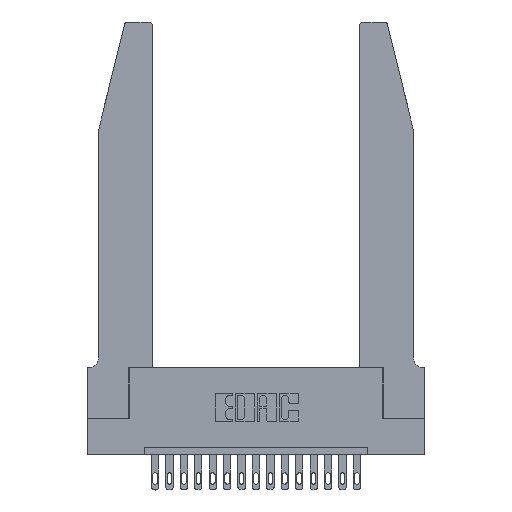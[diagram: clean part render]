
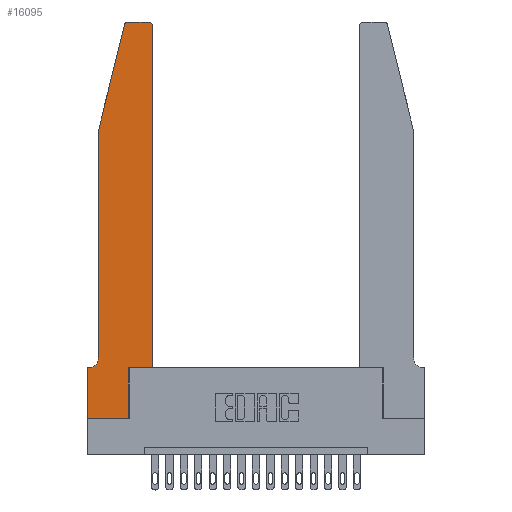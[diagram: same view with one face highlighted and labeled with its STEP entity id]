
A CAD part, top view. The second image highlights one B-rep face of the part: STEP entity #16095.
In plain terms, the highlighted planar face has unit normal (0, 0, 1).
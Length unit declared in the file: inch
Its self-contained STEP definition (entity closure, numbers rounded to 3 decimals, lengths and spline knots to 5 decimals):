
#24 = DIRECTION ( 'NONE',  ( 1., 0., 0. ) ) ;
#91 = DIRECTION ( 'NONE',  ( 0., 1., 0. ) ) ;
#96 = VECTOR ( 'NONE', #12066, 39.37008 ) ;
#188 = VECTOR ( 'NONE', #8749, 39.37008 ) ;
#674 = VECTOR ( 'NONE', #91, 39.37008 ) ;
#808 = CARTESIAN_POINT ( 'NONE',  ( 0.4505, 0.35, 0.37 ) ) ;
#891 = ORIENTED_EDGE ( 'NONE', *, *, #6180, .T. ) ;
#1024 = EDGE_CURVE ( 'NONE', #6409, #7204, #5909, .T. ) ;
#1132 = DIRECTION ( 'NONE',  ( 0., 0., 1. ) ) ;
#1140 = CARTESIAN_POINT ( 'NONE',  ( 0., 0.35, 0.37 ) ) ;
#1428 = VERTEX_POINT ( 'NONE', #13695 ) ;
#1525 = ORIENTED_EDGE ( 'NONE', *, *, #14287, .T. ) ;
#1633 = CARTESIAN_POINT ( 'NONE',  ( 0.2865, 0.35, 0.37 ) ) ;
#1952 = ORIENTED_EDGE ( 'NONE', *, *, #12184, .T. ) ;
#2261 = AXIS2_PLACEMENT_3D ( 'NONE', #11477, #1132, #11677 ) ;
#2593 = CARTESIAN_POINT ( 'NONE',  ( 0.0055, 0.35, 0.37 ) ) ;
#2756 = CIRCLE ( 'NONE', #7343, 0.03 ) ;
#2979 = CARTESIAN_POINT ( 'NONE',  ( 0.0755, 2., 0.37 ) ) ;
#3049 = EDGE_CURVE ( 'NONE', #4441, #1428, #5342, .T. ) ;
#3478 = CARTESIAN_POINT ( 'NONE',  ( 0.0755, 2., 0.37 ) ) ;
#3557 = LINE ( 'NONE', #12129, #8222 ) ;
#3671 = CARTESIAN_POINT ( 'NONE',  ( 0.284, 2.75, 0.37 ) ) ;
#3723 = DIRECTION ( 'NONE',  ( -1., 0., 0. ) ) ;
#3912 = CARTESIAN_POINT ( 'NONE',  ( 0.0755, 2., 0.37 ) ) ;
#3958 = LINE ( 'NONE', #9079, #674 ) ;
#4337 = VERTEX_POINT ( 'NONE', #14523 ) ;
#4441 = VERTEX_POINT ( 'NONE', #6452 ) ;
#4548 = LINE ( 'NONE', #15057, #96 ) ;
#4711 = EDGE_CURVE ( 'NONE', #12307, #4441, #3557, .T. ) ;
#5292 = CARTESIAN_POINT ( 'NONE',  ( 0.2605, 2.75, 0.37 ) ) ;
#5342 = LINE ( 'NONE', #6000, #188 ) ;
#5587 = AXIS2_PLACEMENT_3D ( 'NONE', #15855, #12849, #13053 ) ;
#5701 = ORIENTED_EDGE ( 'NONE', *, *, #3049, .T. ) ;
#5909 = CIRCLE ( 'NONE', #2261, 0.03 ) ;
#6000 = CARTESIAN_POINT ( 'NONE',  ( 0., 0., 0.37 ) ) ;
#6035 = EDGE_CURVE ( 'NONE', #13699, #18647, #12219, .T. ) ;
#6095 = CARTESIAN_POINT ( 'NONE',  ( 0.0755, 0.42, 0.37 ) ) ;
#6180 = EDGE_CURVE ( 'NONE', #18647, #6409, #3958, .T. ) ;
#6409 = VERTEX_POINT ( 'NONE', #8514 ) ;
#6452 = CARTESIAN_POINT ( 'NONE',  ( 0., 0., 0.37 ) ) ;
#7204 = VERTEX_POINT ( 'NONE', #19389 ) ;
#7343 = AXIS2_PLACEMENT_3D ( 'NONE', #9018, #10555, #24 ) ;
#7453 = VECTOR ( 'NONE', #13161, 39.37008 ) ;
#7512 = ORIENTED_EDGE ( 'NONE', *, *, #1024, .T. ) ;
#7542 = ORIENTED_EDGE ( 'NONE', *, *, #15365, .T. ) ;
#7652 = VECTOR ( 'NONE', #3723, 39.37008 ) ;
#7674 = EDGE_CURVE ( 'NONE', #10217, #12307, #13362, .T. ) ;
#7879 = LINE ( 'NONE', #2979, #9294 ) ;
#8222 = VECTOR ( 'NONE', #13640, 39.37008 ) ;
#8514 = CARTESIAN_POINT ( 'NONE',  ( 0.4505, 2.72, 0.37 ) ) ;
#8636 = ORIENTED_EDGE ( 'NONE', *, *, #6035, .T. ) ;
#8657 = VERTEX_POINT ( 'NONE', #3671 ) ;
#8749 = DIRECTION ( 'NONE',  ( 1., 0., 0. ) ) ;
#9018 = CARTESIAN_POINT ( 'NONE',  ( 0.284, 2.72, 0.37 ) ) ;
#9079 = CARTESIAN_POINT ( 'NONE',  ( 0.4505, 0.35, 0.37 ) ) ;
#9294 = VECTOR ( 'NONE', #19417, 39.37008 ) ;
#9900 = DIRECTION ( 'NONE',  ( 1., 0., 0. ) ) ;
#10066 = CARTESIAN_POINT ( 'NONE',  ( 0.0755, 0.35, 0.37 ) ) ;
#10217 = VERTEX_POINT ( 'NONE', #2593 ) ;
#10555 = DIRECTION ( 'NONE',  ( 0., 0., 1. ) ) ;
#10590 = CARTESIAN_POINT ( 'NONE',  ( 0.4505, 0.35, 0.37 ) ) ;
#11477 = CARTESIAN_POINT ( 'NONE',  ( 0.4205, 2.72, 0.37 ) ) ;
#11675 = LINE ( 'NONE', #3912, #14041 ) ;
#11677 = DIRECTION ( 'NONE',  ( 1., 0., 0. ) ) ;
#11908 = VERTEX_POINT ( 'NONE', #6095 ) ;
#12066 = DIRECTION ( 'NONE',  ( 0., 1., 0. ) ) ;
#12129 = CARTESIAN_POINT ( 'NONE',  ( 0., 0., 0.37 ) ) ;
#12184 = EDGE_CURVE ( 'NONE', #11908, #10217, #17732, .T. ) ;
#12219 = LINE ( 'NONE', #808, #17445 ) ;
#12307 = VERTEX_POINT ( 'NONE', #1140 ) ;
#12371 = VERTEX_POINT ( 'NONE', #3478 ) ;
#12660 = ORIENTED_EDGE ( 'NONE', *, *, #4711, .T. ) ;
#12849 = DIRECTION ( 'NONE',  ( 0., 0., 1. ) ) ;
#13053 = DIRECTION ( 'NONE',  ( 1., 0., 0. ) ) ;
#13084 = CARTESIAN_POINT ( 'NONE',  ( 0.0055, 0.42, 0.37 ) ) ;
#13117 = PLANE ( 'NONE',  #5587 ) ;
#13161 = DIRECTION ( 'NONE',  ( -1., 0., 0. ) ) ;
#13362 = LINE ( 'NONE', #10066, #7453 ) ;
#13560 = EDGE_LOOP ( 'NONE', ( #15271, #1525, #18104, #7542, #1952, #19356, #12660, #5701, #14019, #8636, #891, #7512 ) ) ;
#13640 = DIRECTION ( 'NONE',  ( 0., -1., 0. ) ) ;
#13695 = CARTESIAN_POINT ( 'NONE',  ( 0.2865, 0., 0.37 ) ) ;
#13699 = VERTEX_POINT ( 'NONE', #1633 ) ;
#14019 = ORIENTED_EDGE ( 'NONE', *, *, #16375, .T. ) ;
#14041 = VECTOR ( 'NONE', #18888, 39.37008 ) ;
#14253 = FACE_OUTER_BOUND ( 'NONE', #13560, .T. ) ;
#14287 = EDGE_CURVE ( 'NONE', #8657, #4337, #2756, .T. ) ;
#14523 = CARTESIAN_POINT ( 'NONE',  ( 0.25487, 2.72718, 0.37 ) ) ;
#15057 = CARTESIAN_POINT ( 'NONE',  ( 0.2865, 0.35, 0.37 ) ) ;
#15105 = EDGE_CURVE ( 'NONE', #4337, #12371, #11675, .T. ) ;
#15109 = EDGE_CURVE ( 'NONE', #7204, #8657, #15477, .T. ) ;
#15271 = ORIENTED_EDGE ( 'NONE', *, *, #15109, .T. ) ;
#15365 = EDGE_CURVE ( 'NONE', #12371, #11908, #7879, .T. ) ;
#15477 = LINE ( 'NONE', #5292, #7652 ) ;
#15855 = CARTESIAN_POINT ( 'NONE',  ( 0., 0.35, 0.37 ) ) ;
#16007 = DIRECTION ( 'NONE',  ( -1., 0., 0. ) ) ;
#16095 = ADVANCED_FACE ( 'NONE', ( #14253 ), #13117, .T. ) ;
#16375 = EDGE_CURVE ( 'NONE', #1428, #13699, #4548, .T. ) ;
#17084 = AXIS2_PLACEMENT_3D ( 'NONE', #13084, #17344, #16007 ) ;
#17344 = DIRECTION ( 'NONE',  ( 0., 0., -1. ) ) ;
#17445 = VECTOR ( 'NONE', #9900, 39.37008 ) ;
#17732 = CIRCLE ( 'NONE', #17084, 0.07 ) ;
#18104 = ORIENTED_EDGE ( 'NONE', *, *, #15105, .T. ) ;
#18647 = VERTEX_POINT ( 'NONE', #10590 ) ;
#18888 = DIRECTION ( 'NONE',  ( -0.239, -0.971, 0. ) ) ;
#19356 = ORIENTED_EDGE ( 'NONE', *, *, #7674, .T. ) ;
#19389 = CARTESIAN_POINT ( 'NONE',  ( 0.4205, 2.75, 0.37 ) ) ;
#19417 = DIRECTION ( 'NONE',  ( 0., -1., 0. ) ) ;
